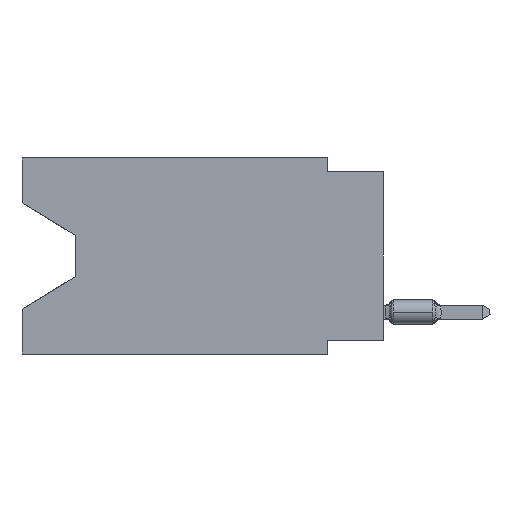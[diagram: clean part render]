
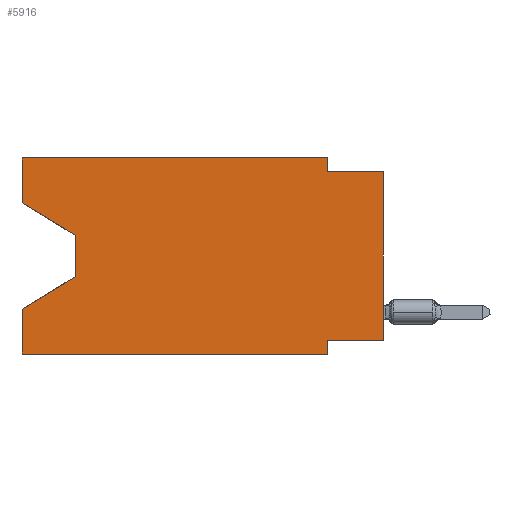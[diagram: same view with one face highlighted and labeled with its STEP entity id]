
A CAD part, left-side view. The second image highlights one B-rep face of the part: STEP entity #5916.
In plain terms, the highlighted planar face has unit normal (-1, 0, 0).
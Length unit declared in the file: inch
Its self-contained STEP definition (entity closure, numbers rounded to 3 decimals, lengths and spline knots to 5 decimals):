
#792 = EDGE_CURVE ( 'NONE', #17769, #11166, #31582, .T. ) ;
#1070 = EDGE_CURVE ( 'NONE', #23132, #23244, #12184, .T. ) ;
#1675 = CARTESIAN_POINT ( 'NONE',  ( 0., 0., -0.325 ) ) ;
#1753 = ORIENTED_EDGE ( 'NONE', *, *, #1070, .F. ) ;
#1892 = DIRECTION ( 'NONE',  ( 0., 0., 1. ) ) ;
#1988 = AXIS2_PLACEMENT_3D ( 'NONE', #26076, #33528, #28952 ) ;
#2652 = DIRECTION ( 'NONE',  ( 0., -1., 0. ) ) ;
#3259 = LINE ( 'NONE', #31290, #31017 ) ;
#3434 = DIRECTION ( 'NONE',  ( 0., 0., 1. ) ) ;
#3999 = VECTOR ( 'NONE', #2652, 39.37008 ) ;
#4406 = LINE ( 'NONE', #1675, #31359 ) ;
#4682 = LINE ( 'NONE', #20831, #3999 ) ;
#4888 = DIRECTION ( 'NONE',  ( 0., -0.855, -0.519 ) ) ;
#5049 = EDGE_CURVE ( 'NONE', #19964, #10181, #31137, .T. ) ;
#5067 = CARTESIAN_POINT ( 'NONE',  ( 0., 0., -0.025 ) ) ;
#5490 = CARTESIAN_POINT ( 'NONE',  ( 0., 0., -0.025 ) ) ;
#5916 = ADVANCED_FACE ( 'NONE', ( #20965 ), #25903, .F. ) ;
#6277 = VECTOR ( 'NONE', #18062, 39.37008 ) ;
#6757 = VERTEX_POINT ( 'NONE', #31543 ) ;
#7049 = ORIENTED_EDGE ( 'NONE', *, *, #13129, .T. ) ;
#7487 = VECTOR ( 'NONE', #28279, 39.37008 ) ;
#7748 = CARTESIAN_POINT ( 'NONE',  ( 0., 0.1, -0.325 ) ) ;
#8998 = DIRECTION ( 'NONE',  ( 0., 1., 0. ) ) ;
#9280 = CARTESIAN_POINT ( 'NONE',  ( 0., 0.645, -0.26975 ) ) ;
#10077 = CARTESIAN_POINT ( 'NONE',  ( 0., 0.55, -0.138 ) ) ;
#10181 = VERTEX_POINT ( 'NONE', #5067 ) ;
#10763 = ORIENTED_EDGE ( 'NONE', *, *, #31634, .T. ) ;
#10778 = VERTEX_POINT ( 'NONE', #7748 ) ;
#11166 = VERTEX_POINT ( 'NONE', #9280 ) ;
#11254 = VECTOR ( 'NONE', #31408, 39.37008 ) ;
#11269 = CARTESIAN_POINT ( 'NONE',  ( 0., 0.645, -0.35 ) ) ;
#11497 = CARTESIAN_POINT ( 'NONE',  ( 0., 0.1, -0.025 ) ) ;
#11593 = EDGE_CURVE ( 'NONE', #6757, #10181, #16875, .T. ) ;
#12184 = LINE ( 'NONE', #22561, #17393 ) ;
#13129 = EDGE_CURVE ( 'NONE', #26940, #27368, #4682, .T. ) ;
#13233 = DIRECTION ( 'NONE',  ( 0., 0.855, -0.519 ) ) ;
#13596 = VECTOR ( 'NONE', #13233, 39.37008 ) ;
#13627 = DIRECTION ( 'NONE',  ( 0., 0., 1. ) ) ;
#14505 = LINE ( 'NONE', #17906, #7487 ) ;
#15074 = VECTOR ( 'NONE', #3434, 39.37008 ) ;
#16766 = EDGE_CURVE ( 'NONE', #25660, #17769, #23332, .T. ) ;
#16875 = LINE ( 'NONE', #27745, #23699 ) ;
#17393 = VECTOR ( 'NONE', #33251, 39.37008 ) ;
#17769 = VERTEX_POINT ( 'NONE', #18700 ) ;
#17906 = CARTESIAN_POINT ( 'NONE',  ( 0., 0.1, -0.35 ) ) ;
#18062 = DIRECTION ( 'NONE',  ( 0., 0., -1. ) ) ;
#18125 = EDGE_CURVE ( 'NONE', #23244, #19964, #21231, .T. ) ;
#18700 = CARTESIAN_POINT ( 'NONE',  ( 0., 0.55, -0.212 ) ) ;
#19822 = CARTESIAN_POINT ( 'NONE',  ( 0., 0.1, -0.35 ) ) ;
#19964 = VERTEX_POINT ( 'NONE', #11497 ) ;
#20188 = CARTESIAN_POINT ( 'NONE',  ( 0., 0.645, -0.08025 ) ) ;
#20831 = CARTESIAN_POINT ( 'NONE',  ( 0., 0.645, -0.35 ) ) ;
#20965 = FACE_OUTER_BOUND ( 'NONE', #30524, .T. ) ;
#21125 = DIRECTION ( 'NONE',  ( 0., -1., 0. ) ) ;
#21231 = LINE ( 'NONE', #29523, #11254 ) ;
#21314 = ORIENTED_EDGE ( 'NONE', *, *, #11593, .T. ) ;
#21398 = EDGE_CURVE ( 'NONE', #31742, #23132, #23664, .T. ) ;
#22431 = CARTESIAN_POINT ( 'NONE',  ( 0., 0.55, -0.138 ) ) ;
#22561 = CARTESIAN_POINT ( 'NONE',  ( 0., 0.645, 0. ) ) ;
#22756 = CARTESIAN_POINT ( 'NONE',  ( 0., 0.645, 0. ) ) ;
#23057 = EDGE_CURVE ( 'NONE', #6757, #10778, #4406, .T. ) ;
#23132 = VERTEX_POINT ( 'NONE', #22756 ) ;
#23244 = VERTEX_POINT ( 'NONE', #25288 ) ;
#23317 = ORIENTED_EDGE ( 'NONE', *, *, #26549, .F. ) ;
#23332 = LINE ( 'NONE', #10077, #6277 ) ;
#23664 = LINE ( 'NONE', #24010, #15074 ) ;
#23699 = VECTOR ( 'NONE', #1892, 39.37008 ) ;
#23955 = CARTESIAN_POINT ( 'NONE',  ( 0., 0.55, -0.212 ) ) ;
#24010 = CARTESIAN_POINT ( 'NONE',  ( 0., 0.645, 0. ) ) ;
#24120 = ORIENTED_EDGE ( 'NONE', *, *, #5049, .F. ) ;
#25005 = ORIENTED_EDGE ( 'NONE', *, *, #32532, .F. ) ;
#25268 = CARTESIAN_POINT ( 'NONE',  ( 0., 0.645, -0.08025 ) ) ;
#25288 = CARTESIAN_POINT ( 'NONE',  ( 0., 0.1, 0. ) ) ;
#25660 = VERTEX_POINT ( 'NONE', #22431 ) ;
#25903 = PLANE ( 'NONE',  #1988 ) ;
#26076 = CARTESIAN_POINT ( 'NONE',  ( 0., 0.645, 0. ) ) ;
#26549 = EDGE_CURVE ( 'NONE', #10778, #27368, #14505, .T. ) ;
#26926 = VECTOR ( 'NONE', #21125, 39.37008 ) ;
#26940 = VERTEX_POINT ( 'NONE', #11269 ) ;
#27368 = VERTEX_POINT ( 'NONE', #19822 ) ;
#27745 = CARTESIAN_POINT ( 'NONE',  ( 0., 0., 0. ) ) ;
#27848 = ORIENTED_EDGE ( 'NONE', *, *, #23057, .F. ) ;
#28279 = DIRECTION ( 'NONE',  ( 0., 0., -1. ) ) ;
#28952 = DIRECTION ( 'NONE',  ( 0., 0., -1. ) ) ;
#29059 = ORIENTED_EDGE ( 'NONE', *, *, #792, .T. ) ;
#29523 = CARTESIAN_POINT ( 'NONE',  ( 0., 0.1, 0. ) ) ;
#29911 = VECTOR ( 'NONE', #4888, 39.37008 ) ;
#30481 = ORIENTED_EDGE ( 'NONE', *, *, #21398, .F. ) ;
#30524 = EDGE_LOOP ( 'NONE', ( #10763, #32930, #29059, #25005, #7049, #23317, #27848, #21314, #24120, #30558, #1753, #30481 ) ) ;
#30558 = ORIENTED_EDGE ( 'NONE', *, *, #18125, .F. ) ;
#31017 = VECTOR ( 'NONE', #13627, 39.37008 ) ;
#31041 = LINE ( 'NONE', #25268, #29911 ) ;
#31137 = LINE ( 'NONE', #5490, #26926 ) ;
#31290 = CARTESIAN_POINT ( 'NONE',  ( 0., 0.645, 0. ) ) ;
#31359 = VECTOR ( 'NONE', #8998, 39.37008 ) ;
#31408 = DIRECTION ( 'NONE',  ( 0., 0., -1. ) ) ;
#31543 = CARTESIAN_POINT ( 'NONE',  ( 0., 0., -0.325 ) ) ;
#31582 = LINE ( 'NONE', #23955, #13596 ) ;
#31634 = EDGE_CURVE ( 'NONE', #31742, #25660, #31041, .T. ) ;
#31742 = VERTEX_POINT ( 'NONE', #20188 ) ;
#32532 = EDGE_CURVE ( 'NONE', #26940, #11166, #3259, .T. ) ;
#32930 = ORIENTED_EDGE ( 'NONE', *, *, #16766, .T. ) ;
#33251 = DIRECTION ( 'NONE',  ( 0., -1., 0. ) ) ;
#33528 = DIRECTION ( 'NONE',  ( 1., 0., 0. ) ) ;
